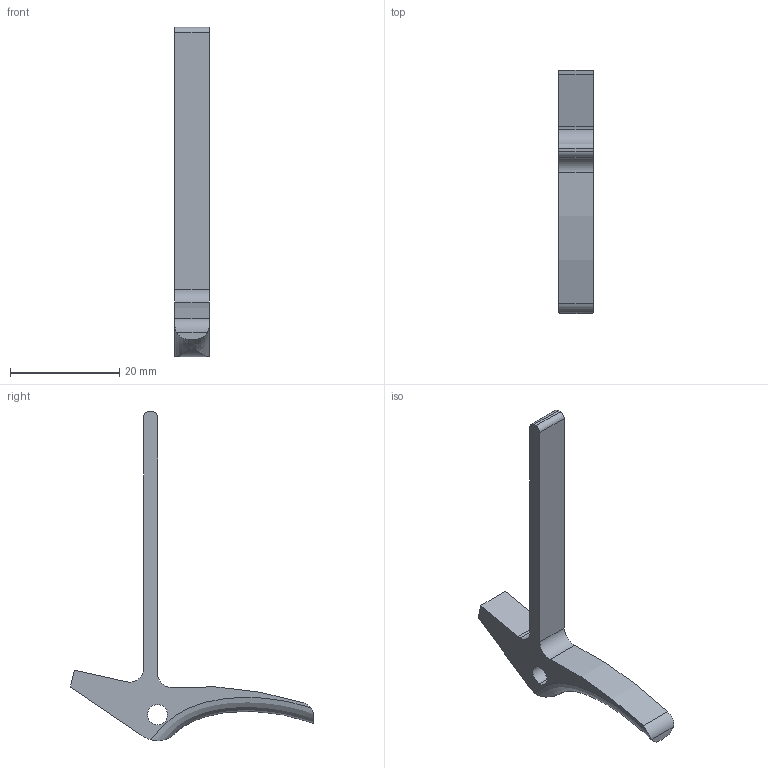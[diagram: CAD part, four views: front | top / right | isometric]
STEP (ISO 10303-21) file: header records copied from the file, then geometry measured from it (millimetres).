
FILE_DESCRIPTION (( 'STEP AP214' ), '1' );
FILE_NAME ('trigger.STEP', '2013-10-27T06:41:39', ( 'Matt' ), ( '' ), 'SwSTEP 2.0', 'SolidWorks 2013', '' );
FILE_SCHEMA (( 'AUTOMOTIVE_DESIGN' ));
Length unit declared in the file: inch
Products named in the file (1): trigger
Bounding box: 6.35 x 44.51 x 60.32 mm (x, y, z)
Volume: 2279.2 mm3; surface area: 1998 mm2
Topology: 1 solids, 1 shells, 22 faces, 60 edges, 40 vertices
Faces by surface type: cylinder 9, plane 9, bspline 4
Entity records: 1209 total; most frequent: CARTESIAN_POINT 624, ORIENTED_EDGE 120, DIRECTION 104, EDGE_CURVE 60, VERTEX_POINT 40, AXIS2_PLACEMENT_3D 37, VECTOR 30, LINE 30
